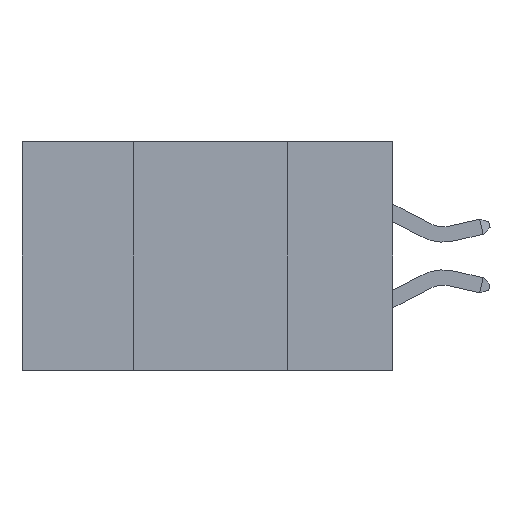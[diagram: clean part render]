
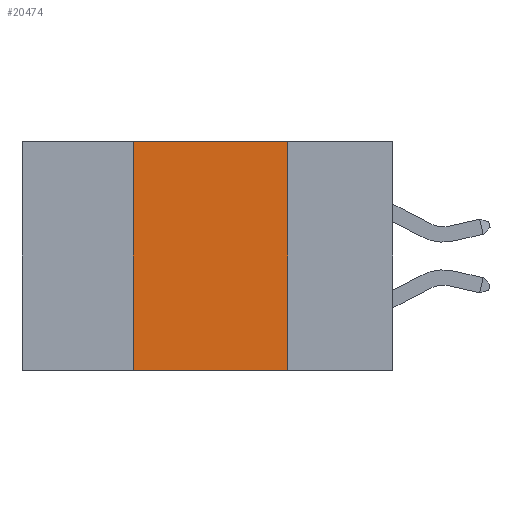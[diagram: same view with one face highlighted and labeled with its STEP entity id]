
A CAD part, left-side view. The second image highlights one B-rep face of the part: STEP entity #20474.
In plain terms, the highlighted planar face has unit normal (-1, 0, 0).
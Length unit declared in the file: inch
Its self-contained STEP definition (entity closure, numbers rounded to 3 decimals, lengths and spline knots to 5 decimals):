
#1085 = DIRECTION ( 'NONE',  ( 0., 0., -1. ) ) ;
#1477 = ORIENTED_EDGE ( 'NONE', *, *, #23785, .T. ) ;
#3343 = CARTESIAN_POINT ( 'NONE',  ( 0., 0.17, 0. ) ) ;
#4096 = CARTESIAN_POINT ( 'NONE',  ( 0., 0.6, 0. ) ) ;
#4603 = ORIENTED_EDGE ( 'NONE', *, *, #25002, .F. ) ;
#4617 = DIRECTION ( 'NONE',  ( 0., 0., 1. ) ) ;
#4700 = LINE ( 'NONE', #9360, #10526 ) ;
#6120 = EDGE_CURVE ( 'NONE', #11560, #14712, #10970, .T. ) ;
#6331 = DIRECTION ( 'NONE',  ( 1., 0., 0. ) ) ;
#9360 = CARTESIAN_POINT ( 'NONE',  ( 0., 0.6, 0. ) ) ;
#9855 = LINE ( 'NONE', #15510, #25567 ) ;
#10526 = VECTOR ( 'NONE', #24329, 39.37008 ) ;
#10970 = LINE ( 'NONE', #3343, #26649 ) ;
#11124 = CARTESIAN_POINT ( 'NONE',  ( 0., 0.42, 0. ) ) ;
#11560 = VERTEX_POINT ( 'NONE', #20118 ) ;
#11585 = CARTESIAN_POINT ( 'NONE',  ( 0., 0.6, -0.37 ) ) ;
#13397 = EDGE_CURVE ( 'NONE', #16355, #27880, #9855, .T. ) ;
#13663 = FACE_OUTER_BOUND ( 'NONE', #13857, .T. ) ;
#13857 = EDGE_LOOP ( 'NONE', ( #24809, #4603, #23826, #1477 ) ) ;
#14712 = VERTEX_POINT ( 'NONE', #19985 ) ;
#15510 = CARTESIAN_POINT ( 'NONE',  ( 0., 0.42, 0. ) ) ;
#16355 = VERTEX_POINT ( 'NONE', #17184 ) ;
#17087 = PLANE ( 'NONE',  #18564 ) ;
#17184 = CARTESIAN_POINT ( 'NONE',  ( 0., 0.42, -0.37 ) ) ;
#18564 = AXIS2_PLACEMENT_3D ( 'NONE', #4096, #6331, #21411 ) ;
#18671 = LINE ( 'NONE', #11585, #24973 ) ;
#19985 = CARTESIAN_POINT ( 'NONE',  ( 0., 0.17, -0.37 ) ) ;
#20118 = CARTESIAN_POINT ( 'NONE',  ( 0., 0.17, 0. ) ) ;
#20474 = ADVANCED_FACE ( 'NONE', ( #13663 ), #17087, .F. ) ;
#21411 = DIRECTION ( 'NONE',  ( 0., 0., -1. ) ) ;
#23785 = EDGE_CURVE ( 'NONE', #16355, #14712, #18671, .T. ) ;
#23826 = ORIENTED_EDGE ( 'NONE', *, *, #13397, .F. ) ;
#24329 = DIRECTION ( 'NONE',  ( 0., -1., 0. ) ) ;
#24809 = ORIENTED_EDGE ( 'NONE', *, *, #6120, .F. ) ;
#24973 = VECTOR ( 'NONE', #26491, 39.37008 ) ;
#25002 = EDGE_CURVE ( 'NONE', #27880, #11560, #4700, .T. ) ;
#25567 = VECTOR ( 'NONE', #4617, 39.37008 ) ;
#26491 = DIRECTION ( 'NONE',  ( 0., -1., 0. ) ) ;
#26649 = VECTOR ( 'NONE', #1085, 39.37008 ) ;
#27880 = VERTEX_POINT ( 'NONE', #11124 ) ;
